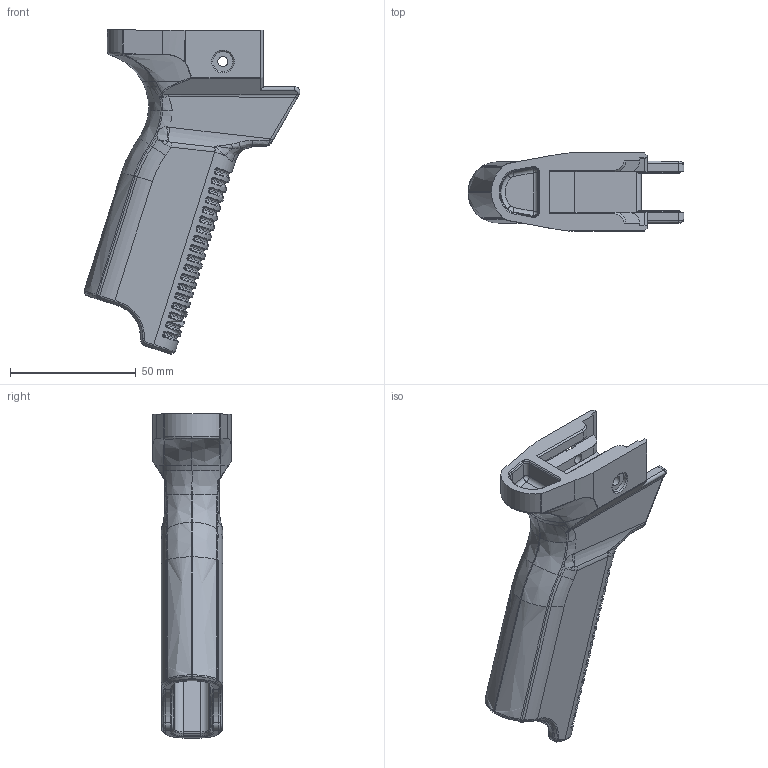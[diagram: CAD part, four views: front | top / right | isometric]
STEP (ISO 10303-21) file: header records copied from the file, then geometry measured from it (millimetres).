
FILE_DESCRIPTION(/* description */ (''),/* implementation_level */ '2;1');
FILE_NAME(/* name */ 'Ridged.step',/* time_stamp */ '2021-09-01T03:01:22-04:00',/* author */ (''),/* organization */ (''),/* preprocessor_version */ 'ST-DEVELOPER v18.1',/* originating_system */ 'Autodesk Translation Framework v10.10.0.1391',/* authorisation */ '');
FILE_SCHEMA (('AUTOMOTIVE_DESIGN { 1 0 10303 214 3 1 1 }'));
Products named in the file (1): Ridged
Bounding box: 85.78 x 31 x 128.74 mm (x, y, z)
Volume: 71696 mm3; surface area: 29651.2 mm2
Topology: 1 solids, 1 shells, 1192 faces, 2876 edges, 1593 vertices
Faces by surface type: bspline 359, cylinder 355, plane 222, torus 214, cone 28, sphere 14
Full cylindrical faces by diameter (mm): 4 x2, 8 x1
Entity records: 49393 total; most frequent: CARTESIAN_POINT 23991, ORIENTED_EDGE 5564, DIRECTION 4947, EDGE_CURVE 2782, AXIS2_PLACEMENT_3D 2025, VERTEX_POINT 1593, EDGE_LOOP 1201, FACE_OUTER_BOUND 1192
